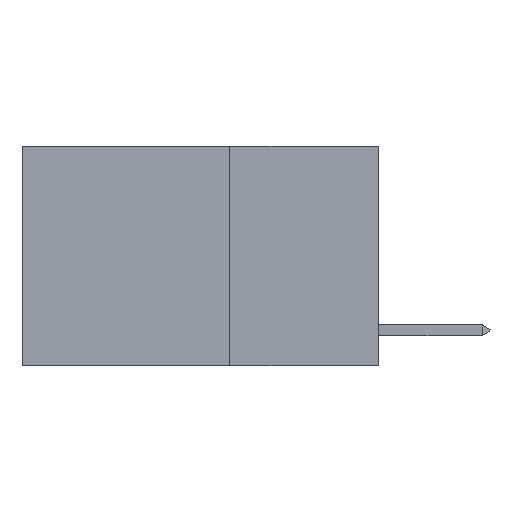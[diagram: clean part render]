
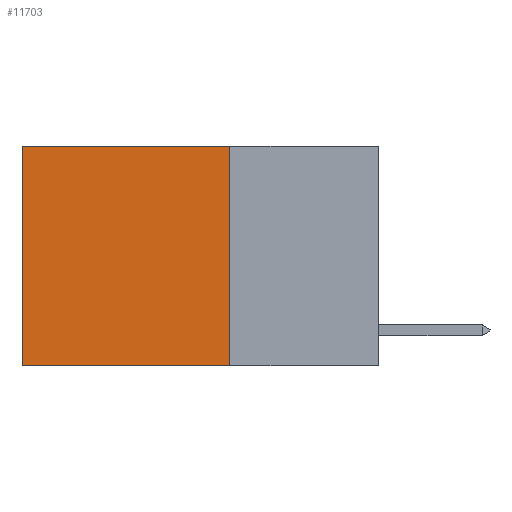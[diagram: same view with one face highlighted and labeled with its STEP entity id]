
A CAD part, left-side view. The second image highlights one B-rep face of the part: STEP entity #11703.
In plain terms, the highlighted planar face has unit normal (-1, 0, 0).
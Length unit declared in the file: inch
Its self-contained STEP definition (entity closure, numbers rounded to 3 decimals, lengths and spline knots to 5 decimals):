
#19 = VECTOR ( 'NONE', #12376, 39.37008 ) ;
#457 = VECTOR ( 'NONE', #14646, 39.37008 ) ;
#874 = CARTESIAN_POINT ( 'NONE',  ( 0.2625, 0.25, 0. ) ) ;
#1062 = ORIENTED_EDGE ( 'NONE', *, *, #18092, .T. ) ;
#2345 = CARTESIAN_POINT ( 'NONE',  ( 0.2625, 0.6, -0.37 ) ) ;
#4186 = DIRECTION ( 'NONE',  ( 0., 0., -1. ) ) ;
#4312 = VERTEX_POINT ( 'NONE', #22397 ) ;
#4505 = FACE_OUTER_BOUND ( 'NONE', #6279, .T. ) ;
#5404 = CARTESIAN_POINT ( 'NONE',  ( 0.2625, 0.6, 0. ) ) ;
#6137 = VERTEX_POINT ( 'NONE', #14762 ) ;
#6231 = CARTESIAN_POINT ( 'NONE',  ( 0.2625, 0.25, -0.37 ) ) ;
#6279 = EDGE_LOOP ( 'NONE', ( #19621, #15551, #10836, #1062 ) ) ;
#6438 = CARTESIAN_POINT ( 'NONE',  ( 0.2625, 0.25, -0.37 ) ) ;
#6558 = LINE ( 'NONE', #6438, #13103 ) ;
#7345 = EDGE_CURVE ( 'NONE', #4312, #20845, #19822, .T. ) ;
#8013 = VECTOR ( 'NONE', #4186, 39.37008 ) ;
#9727 = DIRECTION ( 'NONE',  ( 1., 0., 0. ) ) ;
#10836 = ORIENTED_EDGE ( 'NONE', *, *, #7345, .F. ) ;
#11458 = PLANE ( 'NONE',  #13053 ) ;
#11683 = DIRECTION ( 'NONE',  ( 0., 0., -1. ) ) ;
#11703 = ADVANCED_FACE ( 'NONE', ( #4505 ), #11458, .F. ) ;
#12376 = DIRECTION ( 'NONE',  ( 0., 0., -1. ) ) ;
#13053 = AXIS2_PLACEMENT_3D ( 'NONE', #18416, #9727, #11683 ) ;
#13103 = VECTOR ( 'NONE', #18330, 39.37008 ) ;
#14550 = EDGE_CURVE ( 'NONE', #20845, #19208, #6558, .T. ) ;
#14646 = DIRECTION ( 'NONE',  ( 0., 1., 0. ) ) ;
#14762 = CARTESIAN_POINT ( 'NONE',  ( 0.2625, 0.6, 0. ) ) ;
#14890 = EDGE_CURVE ( 'NONE', #6137, #19208, #17957, .T. ) ;
#15551 = ORIENTED_EDGE ( 'NONE', *, *, #14550, .F. ) ;
#16667 = LINE ( 'NONE', #18307, #457 ) ;
#17957 = LINE ( 'NONE', #5404, #19 ) ;
#18092 = EDGE_CURVE ( 'NONE', #4312, #6137, #16667, .T. ) ;
#18307 = CARTESIAN_POINT ( 'NONE',  ( 0.2625, 0.25, 0. ) ) ;
#18330 = DIRECTION ( 'NONE',  ( 0., 1., 0. ) ) ;
#18416 = CARTESIAN_POINT ( 'NONE',  ( 0.2625, 0.25, 0. ) ) ;
#19208 = VERTEX_POINT ( 'NONE', #2345 ) ;
#19621 = ORIENTED_EDGE ( 'NONE', *, *, #14890, .T. ) ;
#19822 = LINE ( 'NONE', #874, #8013 ) ;
#20845 = VERTEX_POINT ( 'NONE', #6231 ) ;
#22397 = CARTESIAN_POINT ( 'NONE',  ( 0.2625, 0.25, 0. ) ) ;
